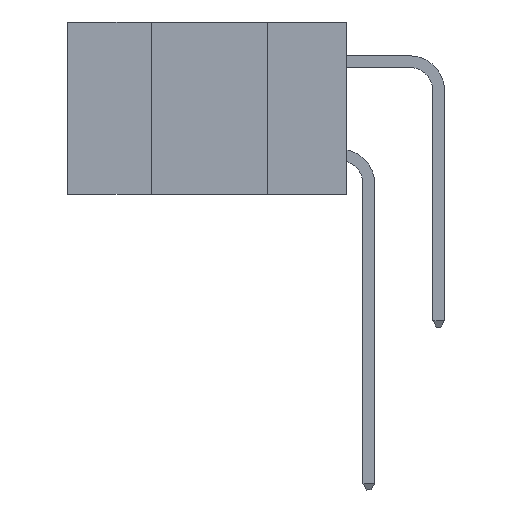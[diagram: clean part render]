
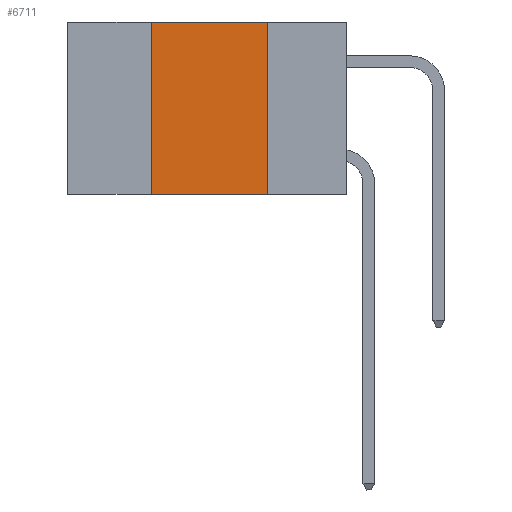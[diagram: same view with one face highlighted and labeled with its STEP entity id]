
A CAD part, left-side view. The second image highlights one B-rep face of the part: STEP entity #6711.
In plain terms, the highlighted planar face has unit normal (-1, 0, 0).
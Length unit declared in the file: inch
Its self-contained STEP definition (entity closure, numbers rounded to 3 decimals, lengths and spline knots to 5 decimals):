
#16 = ORIENTED_EDGE ( 'NONE', *, *, #4537, .F. ) ;
#42 = DIRECTION ( 'NONE',  ( 0., -1., 0. ) ) ;
#357 = LINE ( 'NONE', #13692, #9617 ) ;
#418 = CARTESIAN_POINT ( 'NONE',  ( 0., 0.17, 0. ) ) ;
#1262 = EDGE_CURVE ( 'NONE', #6563, #4084, #13937, .T. ) ;
#1803 = EDGE_CURVE ( 'NONE', #6563, #7076, #12952, .T. ) ;
#3332 = EDGE_LOOP ( 'NONE', ( #4350, #16, #12914, #14055 ) ) ;
#3813 = FACE_OUTER_BOUND ( 'NONE', #3332, .T. ) ;
#4084 = VERTEX_POINT ( 'NONE', #5909 ) ;
#4350 = ORIENTED_EDGE ( 'NONE', *, *, #9965, .F. ) ;
#4537 = EDGE_CURVE ( 'NONE', #7076, #10087, #357, .T. ) ;
#4717 = AXIS2_PLACEMENT_3D ( 'NONE', #5866, #13383, #7033 ) ;
#5115 = DIRECTION ( 'NONE',  ( 0., 0., -1. ) ) ;
#5866 = CARTESIAN_POINT ( 'NONE',  ( 0., 0.6, 0. ) ) ;
#5909 = CARTESIAN_POINT ( 'NONE',  ( 0., 0.17, -0.37 ) ) ;
#6563 = VERTEX_POINT ( 'NONE', #12096 ) ;
#6658 = DIRECTION ( 'NONE',  ( 0., -1., 0. ) ) ;
#6711 = ADVANCED_FACE ( 'NONE', ( #3813 ), #12329, .F. ) ;
#6958 = VECTOR ( 'NONE', #11931, 39.37008 ) ;
#7033 = DIRECTION ( 'NONE',  ( 0., 0., -1. ) ) ;
#7076 = VERTEX_POINT ( 'NONE', #9746 ) ;
#7659 = LINE ( 'NONE', #9450, #9768 ) ;
#8275 = VECTOR ( 'NONE', #6658, 39.37008 ) ;
#9130 = CARTESIAN_POINT ( 'NONE',  ( 0., 0.42, 0. ) ) ;
#9450 = CARTESIAN_POINT ( 'NONE',  ( 0., 0.17, 0. ) ) ;
#9617 = VECTOR ( 'NONE', #42, 39.37008 ) ;
#9746 = CARTESIAN_POINT ( 'NONE',  ( 0., 0.42, 0. ) ) ;
#9768 = VECTOR ( 'NONE', #5115, 39.37008 ) ;
#9965 = EDGE_CURVE ( 'NONE', #10087, #4084, #7659, .T. ) ;
#10087 = VERTEX_POINT ( 'NONE', #418 ) ;
#11931 = DIRECTION ( 'NONE',  ( 0., 0., 1. ) ) ;
#12096 = CARTESIAN_POINT ( 'NONE',  ( 0., 0.42, -0.37 ) ) ;
#12329 = PLANE ( 'NONE',  #4717 ) ;
#12914 = ORIENTED_EDGE ( 'NONE', *, *, #1803, .F. ) ;
#12952 = LINE ( 'NONE', #9130, #6958 ) ;
#13383 = DIRECTION ( 'NONE',  ( 1., 0., 0. ) ) ;
#13692 = CARTESIAN_POINT ( 'NONE',  ( 0., 0.6, 0. ) ) ;
#13937 = LINE ( 'NONE', #14593, #8275 ) ;
#14055 = ORIENTED_EDGE ( 'NONE', *, *, #1262, .T. ) ;
#14593 = CARTESIAN_POINT ( 'NONE',  ( 0., 0.6, -0.37 ) ) ;
